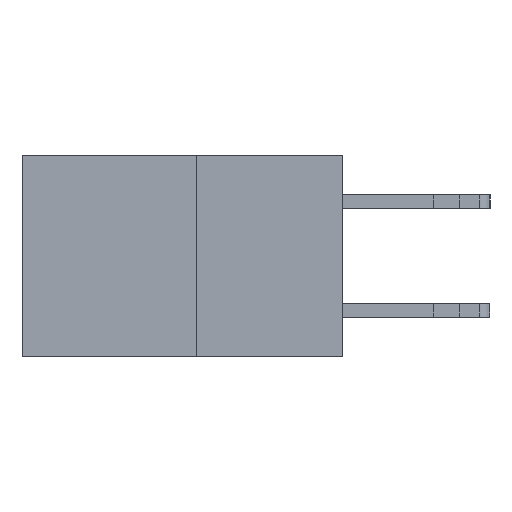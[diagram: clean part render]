
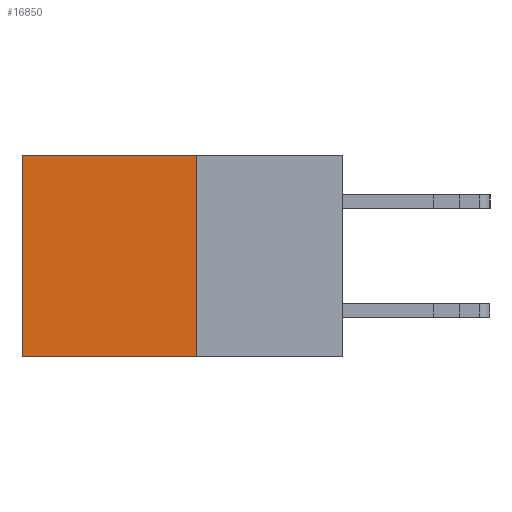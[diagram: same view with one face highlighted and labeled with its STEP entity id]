
A CAD part, left-side view. The second image highlights one B-rep face of the part: STEP entity #16850.
In plain terms, the highlighted planar face has unit normal (-1, 0, 0).
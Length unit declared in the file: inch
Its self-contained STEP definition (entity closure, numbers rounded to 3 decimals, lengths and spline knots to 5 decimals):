
#1105 = DIRECTION ( 'NONE',  ( 0., 1., 0. ) ) ;
#3956 = VECTOR ( 'NONE', #9079, 39.37008 ) ;
#4122 = VERTEX_POINT ( 'NONE', #13300 ) ;
#5145 = ORIENTED_EDGE ( 'NONE', *, *, #23788, .T. ) ;
#5185 = CARTESIAN_POINT ( 'NONE',  ( 0.277, 0.27, -0.37 ) ) ;
#5291 = VECTOR ( 'NONE', #1105, 39.37008 ) ;
#5982 = VECTOR ( 'NONE', #16835, 39.37008 ) ;
#6339 = VERTEX_POINT ( 'NONE', #6770 ) ;
#6406 = ORIENTED_EDGE ( 'NONE', *, *, #7152, .F. ) ;
#6770 = CARTESIAN_POINT ( 'NONE',  ( 0.277, 0.27, -0.37 ) ) ;
#7152 = EDGE_CURVE ( 'NONE', #24619, #6339, #18933, .T. ) ;
#9079 = DIRECTION ( 'NONE',  ( 0., 0., -1. ) ) ;
#9749 = PLANE ( 'NONE',  #14282 ) ;
#9849 = DIRECTION ( 'NONE',  ( 1., 0., 0. ) ) ;
#10999 = EDGE_CURVE ( 'NONE', #6339, #4122, #16936, .T. ) ;
#11488 = DIRECTION ( 'NONE',  ( 0., 0., -1. ) ) ;
#11527 = LINE ( 'NONE', #14777, #5982 ) ;
#12116 = ORIENTED_EDGE ( 'NONE', *, *, #22392, .T. ) ;
#12365 = CARTESIAN_POINT ( 'NONE',  ( 0.277, 0.59, 0. ) ) ;
#13300 = CARTESIAN_POINT ( 'NONE',  ( 0.277, 0.59, -0.37 ) ) ;
#14282 = AXIS2_PLACEMENT_3D ( 'NONE', #22038, #9849, #24065 ) ;
#14777 = CARTESIAN_POINT ( 'NONE',  ( 0.277, 0.27, 0. ) ) ;
#14784 = VECTOR ( 'NONE', #11488, 39.37008 ) ;
#15584 = LINE ( 'NONE', #19256, #3956 ) ;
#16835 = DIRECTION ( 'NONE',  ( 0., 1., 0. ) ) ;
#16850 = ADVANCED_FACE ( 'NONE', ( #25083 ), #9749, .F. ) ;
#16936 = LINE ( 'NONE', #21606, #5291 ) ;
#18933 = LINE ( 'NONE', #5185, #14784 ) ;
#19256 = CARTESIAN_POINT ( 'NONE',  ( 0.277, 0.59, -0.37 ) ) ;
#20548 = ORIENTED_EDGE ( 'NONE', *, *, #10999, .F. ) ;
#21086 = VERTEX_POINT ( 'NONE', #12365 ) ;
#21606 = CARTESIAN_POINT ( 'NONE',  ( 0.277, 0.27, -0.37 ) ) ;
#21688 = CARTESIAN_POINT ( 'NONE',  ( 0.277, 0.27, 0. ) ) ;
#22038 = CARTESIAN_POINT ( 'NONE',  ( 0.277, 0.27, -0.37 ) ) ;
#22107 = EDGE_LOOP ( 'NONE', ( #5145, #20548, #6406, #12116 ) ) ;
#22392 = EDGE_CURVE ( 'NONE', #24619, #21086, #11527, .T. ) ;
#23788 = EDGE_CURVE ( 'NONE', #21086, #4122, #15584, .T. ) ;
#24065 = DIRECTION ( 'NONE',  ( 0., 0., -1. ) ) ;
#24619 = VERTEX_POINT ( 'NONE', #21688 ) ;
#25083 = FACE_OUTER_BOUND ( 'NONE', #22107, .T. ) ;
